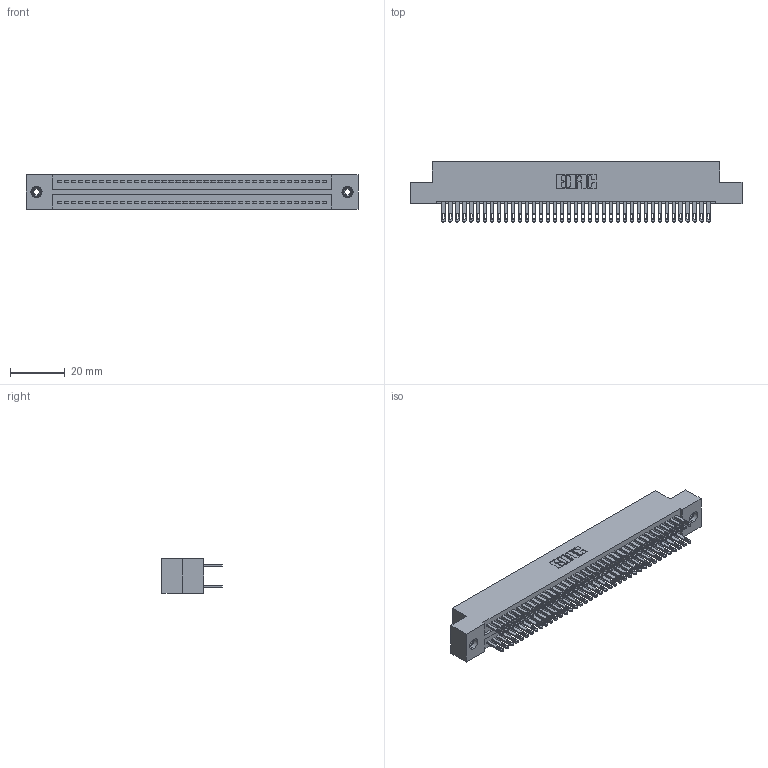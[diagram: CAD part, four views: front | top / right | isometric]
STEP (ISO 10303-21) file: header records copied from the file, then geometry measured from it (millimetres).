
FILE_DESCRIPTION (( 'STEP AP203' ), '1' );
FILE_NAME ('325-078-500-208.STEP', '2020-02-25T04:24:52', ( '' ), ( '' ), 'SwSTEP 2.0', 'SolidWorks 2016', '' );
FILE_SCHEMA (( 'CONFIG_CONTROL_DESIGN' ));
Length unit declared in the file: inch
Products named in the file (4): 325-292-001_325-293-100; 345-250-001_345-250-003-102; 325-078-500-208; 325 Part_TI
Assembly tree (81 placements, depth 2):
  325-078-500-208
    325 Part_TI
    325-292-001_325-293-100  x78
    345-250-001_345-250-003-102  x2
Bounding box: 120.78 x 21.84 x 12.45 mm (x, y, z)
Volume: 15796.7 mm3; surface area: 19877.9 mm2
Topology: 81 solids, 81 shells, 3918 faces, 11913 edges, 7934 vertices
Faces by surface type: plane 2442, cylinder 1460, cone 12, torus 4
Entity records: 26594 total; most frequent: CARTESIAN_POINT 4393, ORIENTED_EDGE 4322, DIRECTION 3791, EDGE_CURVE 2161, VECTOR 2009, LINE 2009, VERTEX_POINT 1436, AXIS2_PLACEMENT_3D 891
